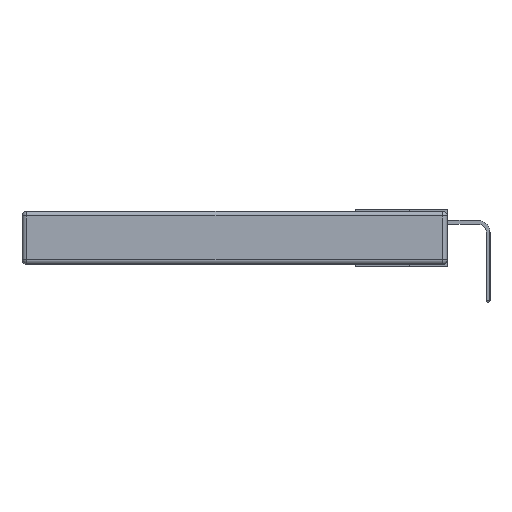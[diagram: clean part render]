
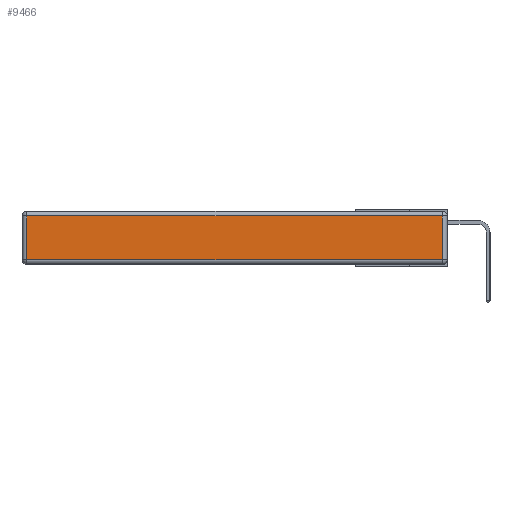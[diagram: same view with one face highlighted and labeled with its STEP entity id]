
A CAD part, left-side view. The second image highlights one B-rep face of the part: STEP entity #9466.
In plain terms, the highlighted planar face has unit normal (-1, 0, 0).
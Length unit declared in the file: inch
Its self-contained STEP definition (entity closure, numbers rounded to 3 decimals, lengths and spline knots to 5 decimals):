
#111 = EDGE_CURVE ( 'NONE', #5718, #3888, #5736, .T. ) ;
#628 = ORIENTED_EDGE ( 'NONE', *, *, #8911, .T. ) ;
#1487 = CARTESIAN_POINT ( 'NONE',  ( 0., 0.03, -0.343 ) ) ;
#1766 = CARTESIAN_POINT ( 'NONE',  ( 0., 0., -0.313 ) ) ;
#2036 = CARTESIAN_POINT ( 'NONE',  ( 0., 0.03, -0.313 ) ) ;
#2912 = VECTOR ( 'NONE', #9291, 39.37008 ) ;
#3268 = ORIENTED_EDGE ( 'NONE', *, *, #4250, .T. ) ;
#3700 = DIRECTION ( 'NONE',  ( 0., -1., 0. ) ) ;
#3888 = VERTEX_POINT ( 'NONE', #9219 ) ;
#3893 = VECTOR ( 'NONE', #5778, 39.37008 ) ;
#4038 = VERTEX_POINT ( 'NONE', #7870 ) ;
#4085 = VERTEX_POINT ( 'NONE', #2036 ) ;
#4250 = EDGE_CURVE ( 'NONE', #4085, #5718, #10974, .T. ) ;
#4815 = CARTESIAN_POINT ( 'NONE',  ( 0., 0.03, -0.03 ) ) ;
#4961 = CARTESIAN_POINT ( 'NONE',  ( 0., 2.75, -0.03 ) ) ;
#5718 = VERTEX_POINT ( 'NONE', #4815 ) ;
#5736 = LINE ( 'NONE', #4961, #9691 ) ;
#5778 = DIRECTION ( 'NONE',  ( 0., 0., -1. ) ) ;
#6208 = LINE ( 'NONE', #8581, #3893 ) ;
#6922 = DIRECTION ( 'NONE',  ( 0., 1., 0. ) ) ;
#6955 = CARTESIAN_POINT ( 'NONE',  ( 0., 0., -0.343 ) ) ;
#7870 = CARTESIAN_POINT ( 'NONE',  ( 0., 2.72, -0.313 ) ) ;
#8581 = CARTESIAN_POINT ( 'NONE',  ( 0., 2.72, -0.343 ) ) ;
#8790 = DIRECTION ( 'NONE',  ( -1., 0., 0. ) ) ;
#8911 = EDGE_CURVE ( 'NONE', #3888, #4038, #6208, .T. ) ;
#9219 = CARTESIAN_POINT ( 'NONE',  ( 0., 2.72, -0.03 ) ) ;
#9291 = DIRECTION ( 'NONE',  ( 0., 0., 1. ) ) ;
#9359 = LINE ( 'NONE', #1766, #10283 ) ;
#9466 = ADVANCED_FACE ( 'NONE', ( #12549 ), #10877, .T. ) ;
#9535 = AXIS2_PLACEMENT_3D ( 'NONE', #6955, #8790, #10746 ) ;
#9691 = VECTOR ( 'NONE', #6922, 39.37008 ) ;
#10283 = VECTOR ( 'NONE', #3700, 39.37008 ) ;
#10746 = DIRECTION ( 'NONE',  ( 0., 0., 1. ) ) ;
#10877 = PLANE ( 'NONE',  #9535 ) ;
#10974 = LINE ( 'NONE', #1487, #2912 ) ;
#11002 = EDGE_CURVE ( 'NONE', #4038, #4085, #9359, .T. ) ;
#11459 = ORIENTED_EDGE ( 'NONE', *, *, #11002, .T. ) ;
#11699 = ORIENTED_EDGE ( 'NONE', *, *, #111, .T. ) ;
#11876 = EDGE_LOOP ( 'NONE', ( #11459, #3268, #11699, #628 ) ) ;
#12549 = FACE_OUTER_BOUND ( 'NONE', #11876, .T. ) ;
